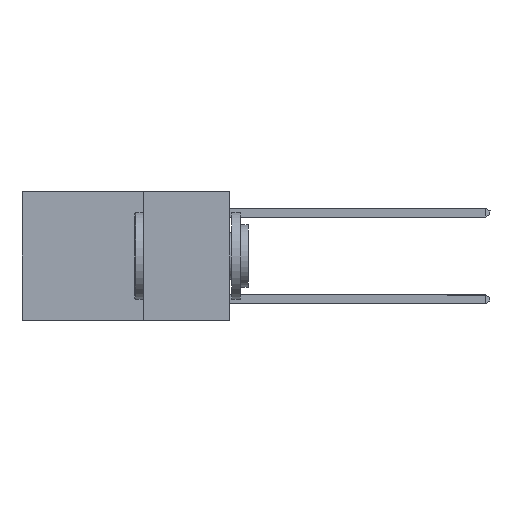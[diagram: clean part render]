
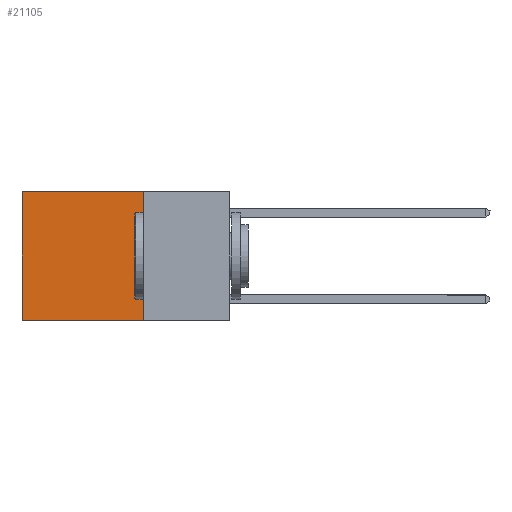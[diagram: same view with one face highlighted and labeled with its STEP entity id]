
A CAD part, left-side view. The second image highlights one B-rep face of the part: STEP entity #21105.
In plain terms, the highlighted planar face has unit normal (-1, 0, 0).
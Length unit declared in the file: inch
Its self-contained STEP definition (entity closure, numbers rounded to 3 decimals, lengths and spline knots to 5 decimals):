
#247 = EDGE_CURVE ( 'NONE', #9828, #15726, #12910, .T. ) ;
#1880 = CARTESIAN_POINT ( 'NONE',  ( 0.2625, 0.25, 0. ) ) ;
#2080 = CARTESIAN_POINT ( 'NONE',  ( 0.2625, 0.6, -0.37 ) ) ;
#2360 = DIRECTION ( 'NONE',  ( 1., 0., 0. ) ) ;
#4517 = LINE ( 'NONE', #1880, #14949 ) ;
#5822 = VERTEX_POINT ( 'NONE', #2080 ) ;
#6908 = CARTESIAN_POINT ( 'NONE',  ( 0.2625, 0.25, 0. ) ) ;
#7576 = CARTESIAN_POINT ( 'NONE',  ( 0.2625, 0.6, 0. ) ) ;
#7939 = VERTEX_POINT ( 'NONE', #23861 ) ;
#8746 = EDGE_CURVE ( 'NONE', #7939, #5822, #22153, .T. ) ;
#9186 = LINE ( 'NONE', #18051, #13503 ) ;
#9828 = VERTEX_POINT ( 'NONE', #6908 ) ;
#11092 = CARTESIAN_POINT ( 'NONE',  ( 0.2625, 0.25, -0.37 ) ) ;
#12575 = DIRECTION ( 'NONE',  ( 0., 1., 0. ) ) ;
#12910 = LINE ( 'NONE', #13354, #17231 ) ;
#12964 = DIRECTION ( 'NONE',  ( 0., 1., 0. ) ) ;
#13354 = CARTESIAN_POINT ( 'NONE',  ( 0.2625, 0.25, 0. ) ) ;
#13429 = CARTESIAN_POINT ( 'NONE',  ( 0.2625, 0.25, 0. ) ) ;
#13478 = EDGE_LOOP ( 'NONE', ( #20161, #22502, #18921, #19676 ) ) ;
#13503 = VECTOR ( 'NONE', #12575, 39.37008 ) ;
#14949 = VECTOR ( 'NONE', #12964, 39.37008 ) ;
#15279 = DIRECTION ( 'NONE',  ( 0., 0., -1. ) ) ;
#15726 = VERTEX_POINT ( 'NONE', #11092 ) ;
#16663 = VECTOR ( 'NONE', #22357, 39.37008 ) ;
#17147 = DIRECTION ( 'NONE',  ( 0., 0., -1. ) ) ;
#17231 = VECTOR ( 'NONE', #17147, 39.37008 ) ;
#18051 = CARTESIAN_POINT ( 'NONE',  ( 0.2625, 0.25, -0.37 ) ) ;
#18911 = PLANE ( 'NONE',  #19983 ) ;
#18921 = ORIENTED_EDGE ( 'NONE', *, *, #247, .F. ) ;
#19676 = ORIENTED_EDGE ( 'NONE', *, *, #22905, .T. ) ;
#19983 = AXIS2_PLACEMENT_3D ( 'NONE', #13429, #2360, #15279 ) ;
#20161 = ORIENTED_EDGE ( 'NONE', *, *, #8746, .T. ) ;
#21105 = ADVANCED_FACE ( 'NONE', ( #22613 ), #18911, .F. ) ;
#22153 = LINE ( 'NONE', #7576, #16663 ) ;
#22357 = DIRECTION ( 'NONE',  ( 0., 0., -1. ) ) ;
#22502 = ORIENTED_EDGE ( 'NONE', *, *, #23174, .F. ) ;
#22613 = FACE_OUTER_BOUND ( 'NONE', #13478, .T. ) ;
#22905 = EDGE_CURVE ( 'NONE', #9828, #7939, #4517, .T. ) ;
#23174 = EDGE_CURVE ( 'NONE', #15726, #5822, #9186, .T. ) ;
#23861 = CARTESIAN_POINT ( 'NONE',  ( 0.2625, 0.6, 0. ) ) ;
